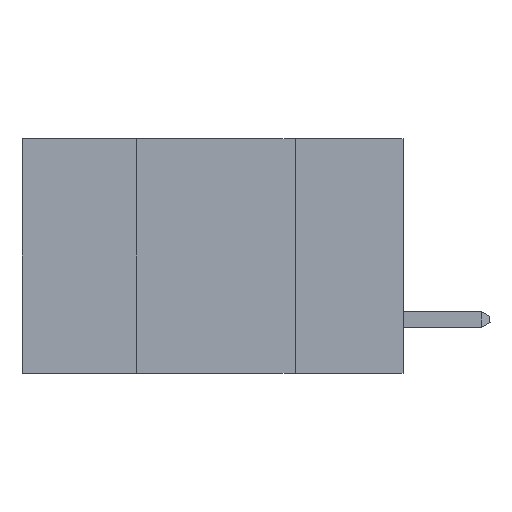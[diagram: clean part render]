
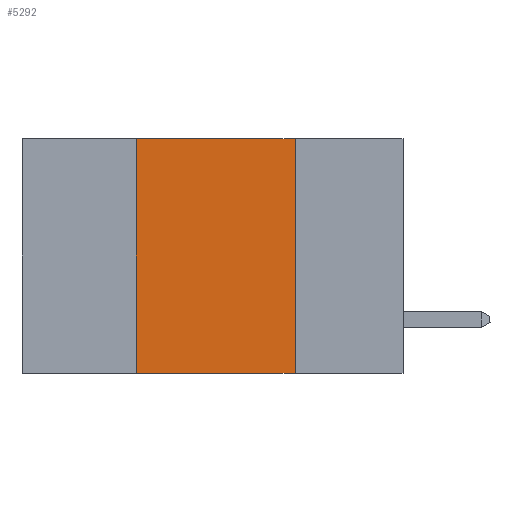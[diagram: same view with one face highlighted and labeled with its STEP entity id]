
A CAD part, left-side view. The second image highlights one B-rep face of the part: STEP entity #5292.
In plain terms, the highlighted planar face has unit normal (-1, 0, 0).
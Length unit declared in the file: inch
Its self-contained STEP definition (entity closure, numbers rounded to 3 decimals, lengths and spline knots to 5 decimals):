
#270 = VECTOR ( 'NONE', #8541, 39.37008 ) ;
#395 = VERTEX_POINT ( 'NONE', #2350 ) ;
#1030 = ORIENTED_EDGE ( 'NONE', *, *, #9232, .F. ) ;
#1632 = DIRECTION ( 'NONE',  ( 1., 0., 0. ) ) ;
#1911 = ORIENTED_EDGE ( 'NONE', *, *, #10034, .T. ) ;
#2320 = LINE ( 'NONE', #2390, #4333 ) ;
#2350 = CARTESIAN_POINT ( 'NONE',  ( 0., 0.42, 0. ) ) ;
#2390 = CARTESIAN_POINT ( 'NONE',  ( 0., 0.6, 0. ) ) ;
#3220 = VECTOR ( 'NONE', #5074, 39.37008 ) ;
#3563 = CARTESIAN_POINT ( 'NONE',  ( 0., 0.17, 0. ) ) ;
#4055 = VERTEX_POINT ( 'NONE', #11430 ) ;
#4137 = CARTESIAN_POINT ( 'NONE',  ( 0., 0.42, 0. ) ) ;
#4333 = VECTOR ( 'NONE', #10722, 39.37008 ) ;
#4711 = LINE ( 'NONE', #11490, #8611 ) ;
#4772 = EDGE_CURVE ( 'NONE', #395, #5198, #2320, .T. ) ;
#4974 = CARTESIAN_POINT ( 'NONE',  ( 0., 0.17, -0.37 ) ) ;
#5074 = DIRECTION ( 'NONE',  ( 0., 0., 1. ) ) ;
#5198 = VERTEX_POINT ( 'NONE', #3563 ) ;
#5292 = ADVANCED_FACE ( 'NONE', ( #6637 ), #10917, .F. ) ;
#5457 = EDGE_LOOP ( 'NONE', ( #1030, #8280, #9474, #1911 ) ) ;
#6162 = EDGE_CURVE ( 'NONE', #4055, #395, #8988, .T. ) ;
#6637 = FACE_OUTER_BOUND ( 'NONE', #5457, .T. ) ;
#6741 = VERTEX_POINT ( 'NONE', #4974 ) ;
#7978 = AXIS2_PLACEMENT_3D ( 'NONE', #9949, #1632, #9166 ) ;
#8280 = ORIENTED_EDGE ( 'NONE', *, *, #4772, .F. ) ;
#8541 = DIRECTION ( 'NONE',  ( 0., 0., -1. ) ) ;
#8611 = VECTOR ( 'NONE', #9643, 39.37008 ) ;
#8622 = LINE ( 'NONE', #9463, #270 ) ;
#8988 = LINE ( 'NONE', #4137, #3220 ) ;
#9166 = DIRECTION ( 'NONE',  ( 0., 0., -1. ) ) ;
#9232 = EDGE_CURVE ( 'NONE', #5198, #6741, #8622, .T. ) ;
#9463 = CARTESIAN_POINT ( 'NONE',  ( 0., 0.17, 0. ) ) ;
#9474 = ORIENTED_EDGE ( 'NONE', *, *, #6162, .F. ) ;
#9643 = DIRECTION ( 'NONE',  ( 0., -1., 0. ) ) ;
#9949 = CARTESIAN_POINT ( 'NONE',  ( 0., 0.6, 0. ) ) ;
#10034 = EDGE_CURVE ( 'NONE', #4055, #6741, #4711, .T. ) ;
#10722 = DIRECTION ( 'NONE',  ( 0., -1., 0. ) ) ;
#10917 = PLANE ( 'NONE',  #7978 ) ;
#11430 = CARTESIAN_POINT ( 'NONE',  ( 0., 0.42, -0.37 ) ) ;
#11490 = CARTESIAN_POINT ( 'NONE',  ( 0., 0.6, -0.37 ) ) ;
